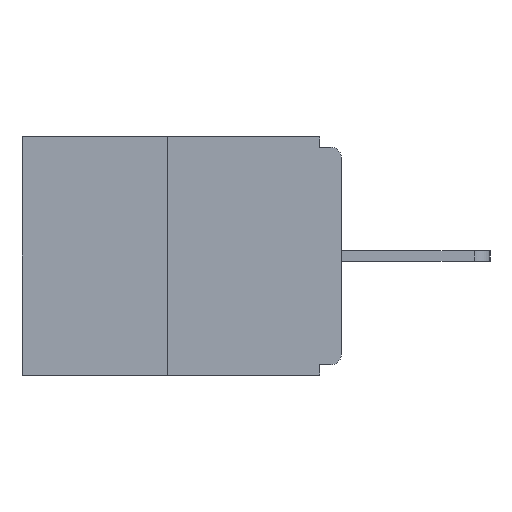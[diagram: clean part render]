
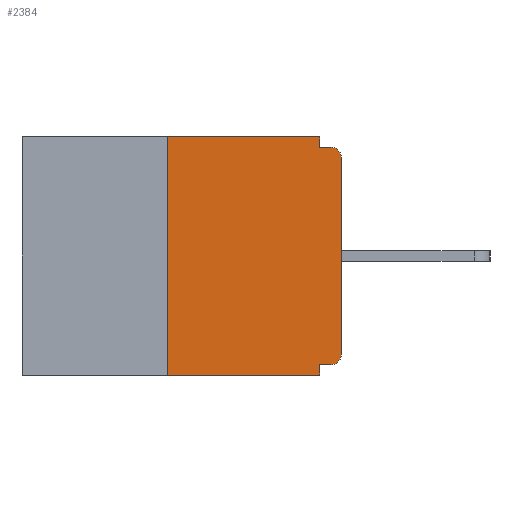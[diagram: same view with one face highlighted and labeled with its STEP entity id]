
A CAD part, left-side view. The second image highlights one B-rep face of the part: STEP entity #2384.
In plain terms, the highlighted planar face has unit normal (-1, 0, 0).
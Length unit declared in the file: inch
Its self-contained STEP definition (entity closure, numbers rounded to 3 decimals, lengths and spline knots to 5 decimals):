
#44 = CARTESIAN_POINT ( 'NONE',  ( 0., 0.031, -0.343 ) ) ;
#167 = VERTEX_POINT ( 'NONE', #15260 ) ;
#539 = DIRECTION ( 'NONE',  ( 0., -1., 0. ) ) ;
#623 = EDGE_CURVE ( 'NONE', #10151, #7984, #14113, .T. ) ;
#648 = EDGE_CURVE ( 'NONE', #14368, #13361, #1942, .T. ) ;
#766 = VERTEX_POINT ( 'NONE', #4637 ) ;
#947 = VERTEX_POINT ( 'NONE', #9393 ) ;
#999 = CIRCLE ( 'NONE', #16829, 0.015 ) ;
#1467 = VECTOR ( 'NONE', #17111, 39.37008 ) ;
#1942 = LINE ( 'NONE', #15775, #1467 ) ;
#2230 = ORIENTED_EDGE ( 'NONE', *, *, #623, .T. ) ;
#2384 = ADVANCED_FACE ( 'NONE', ( #9178 ), #8405, .F. ) ;
#3849 = DIRECTION ( 'NONE',  ( 0., 0., -1. ) ) ;
#4098 = EDGE_LOOP ( 'NONE', ( #8129, #12097, #4496, #8587, #4979, #16843, #13931, #2230, #6925, #14832 ) ) ;
#4496 = ORIENTED_EDGE ( 'NONE', *, *, #6322, .T. ) ;
#4577 = LINE ( 'NONE', #44, #11708 ) ;
#4637 = CARTESIAN_POINT ( 'NONE',  ( 0., 0.015, -0.328 ) ) ;
#4756 = EDGE_CURVE ( 'NONE', #947, #7984, #17838, .T. ) ;
#4979 = ORIENTED_EDGE ( 'NONE', *, *, #18156, .F. ) ;
#5129 = CARTESIAN_POINT ( 'NONE',  ( 0., 0., -0.313 ) ) ;
#5465 = CARTESIAN_POINT ( 'NONE',  ( 0., 0., -0.015 ) ) ;
#5515 = DIRECTION ( 'NONE',  ( -1., 0., 0. ) ) ;
#6079 = EDGE_CURVE ( 'NONE', #9471, #10151, #7489, .T. ) ;
#6322 = EDGE_CURVE ( 'NONE', #14368, #8685, #7713, .T. ) ;
#6344 = DIRECTION ( 'NONE',  ( 0., 0., -1. ) ) ;
#6566 = CARTESIAN_POINT ( 'NONE',  ( 0., 0.031, 0. ) ) ;
#6803 = CARTESIAN_POINT ( 'NONE',  ( 0., 0., -0.03 ) ) ;
#6925 = ORIENTED_EDGE ( 'NONE', *, *, #4756, .F. ) ;
#7489 = LINE ( 'NONE', #17467, #10971 ) ;
#7646 = CARTESIAN_POINT ( 'NONE',  ( 0., 0.25, 0. ) ) ;
#7713 = LINE ( 'NONE', #15084, #11187 ) ;
#7984 = VERTEX_POINT ( 'NONE', #13227 ) ;
#8129 = ORIENTED_EDGE ( 'NONE', *, *, #18732, .F. ) ;
#8405 = PLANE ( 'NONE',  #13386 ) ;
#8587 = ORIENTED_EDGE ( 'NONE', *, *, #13481, .F. ) ;
#8685 = VERTEX_POINT ( 'NONE', #19326 ) ;
#9178 = FACE_OUTER_BOUND ( 'NONE', #4098, .T. ) ;
#9393 = CARTESIAN_POINT ( 'NONE',  ( 0., 0.031, -0.015 ) ) ;
#9471 = VERTEX_POINT ( 'NONE', #5129 ) ;
#9526 = DIRECTION ( 'NONE',  ( 0., -1., 0. ) ) ;
#10151 = VERTEX_POINT ( 'NONE', #6803 ) ;
#10216 = DIRECTION ( 'NONE',  ( 0., 0., 1. ) ) ;
#10243 = EDGE_CURVE ( 'NONE', #766, #9471, #999, .T. ) ;
#10971 = VECTOR ( 'NONE', #10216, 39.37008 ) ;
#11049 = CARTESIAN_POINT ( 'NONE',  ( 0., 0.46, 0. ) ) ;
#11187 = VECTOR ( 'NONE', #19380, 39.37008 ) ;
#11221 = VECTOR ( 'NONE', #17118, 39.37008 ) ;
#11341 = LINE ( 'NONE', #12944, #11830 ) ;
#11708 = VECTOR ( 'NONE', #6344, 39.37008 ) ;
#11830 = VECTOR ( 'NONE', #3849, 39.37008 ) ;
#12097 = ORIENTED_EDGE ( 'NONE', *, *, #648, .F. ) ;
#12810 = DIRECTION ( 'NONE',  ( 0., 0., -1. ) ) ;
#12919 = VERTEX_POINT ( 'NONE', #6566 ) ;
#12944 = CARTESIAN_POINT ( 'NONE',  ( 0., 0.031, 0. ) ) ;
#13125 = VECTOR ( 'NONE', #539, 39.37008 ) ;
#13227 = CARTESIAN_POINT ( 'NONE',  ( 0., 0.015, -0.015 ) ) ;
#13361 = VERTEX_POINT ( 'NONE', #7646 ) ;
#13386 = AXIS2_PLACEMENT_3D ( 'NONE', #11049, #13943, #12810 ) ;
#13481 = EDGE_CURVE ( 'NONE', #167, #8685, #4577, .T. ) ;
#13922 = CARTESIAN_POINT ( 'NONE',  ( 0., 0.015, -0.03 ) ) ;
#13931 = ORIENTED_EDGE ( 'NONE', *, *, #6079, .T. ) ;
#13943 = DIRECTION ( 'NONE',  ( 1., 0., 0. ) ) ;
#14035 = VECTOR ( 'NONE', #9526, 39.37008 ) ;
#14113 = CIRCLE ( 'NONE', #15865, 0.015 ) ;
#14368 = VERTEX_POINT ( 'NONE', #18292 ) ;
#14496 = CARTESIAN_POINT ( 'NONE',  ( 0., 0.015, -0.313 ) ) ;
#14832 = ORIENTED_EDGE ( 'NONE', *, *, #15741, .F. ) ;
#15084 = CARTESIAN_POINT ( 'NONE',  ( 0., 0.46, -0.343 ) ) ;
#15260 = CARTESIAN_POINT ( 'NONE',  ( 0., 0.031, -0.328 ) ) ;
#15682 = CARTESIAN_POINT ( 'NONE',  ( 0., 0., -0.328 ) ) ;
#15741 = EDGE_CURVE ( 'NONE', #12919, #947, #11341, .T. ) ;
#15775 = CARTESIAN_POINT ( 'NONE',  ( 0., 0.25, 0. ) ) ;
#15865 = AXIS2_PLACEMENT_3D ( 'NONE', #13922, #16880, #16451 ) ;
#15920 = DIRECTION ( 'NONE',  ( 0., 0., -1. ) ) ;
#16451 = DIRECTION ( 'NONE',  ( 0., 0., -1. ) ) ;
#16829 = AXIS2_PLACEMENT_3D ( 'NONE', #14496, #5515, #15920 ) ;
#16843 = ORIENTED_EDGE ( 'NONE', *, *, #10243, .T. ) ;
#16880 = DIRECTION ( 'NONE',  ( -1., 0., 0. ) ) ;
#16921 = LINE ( 'NONE', #18512, #13125 ) ;
#17111 = DIRECTION ( 'NONE',  ( 0., 0., 1. ) ) ;
#17118 = DIRECTION ( 'NONE',  ( 0., 1., 0. ) ) ;
#17467 = CARTESIAN_POINT ( 'NONE',  ( 0., 0., 0. ) ) ;
#17838 = LINE ( 'NONE', #5465, #14035 ) ;
#18156 = EDGE_CURVE ( 'NONE', #766, #167, #18892, .T. ) ;
#18292 = CARTESIAN_POINT ( 'NONE',  ( 0., 0.25, -0.343 ) ) ;
#18512 = CARTESIAN_POINT ( 'NONE',  ( 0., 0.46, 0. ) ) ;
#18732 = EDGE_CURVE ( 'NONE', #13361, #12919, #16921, .T. ) ;
#18892 = LINE ( 'NONE', #15682, #11221 ) ;
#19326 = CARTESIAN_POINT ( 'NONE',  ( 0., 0.031, -0.343 ) ) ;
#19380 = DIRECTION ( 'NONE',  ( 0., -1., 0. ) ) ;
